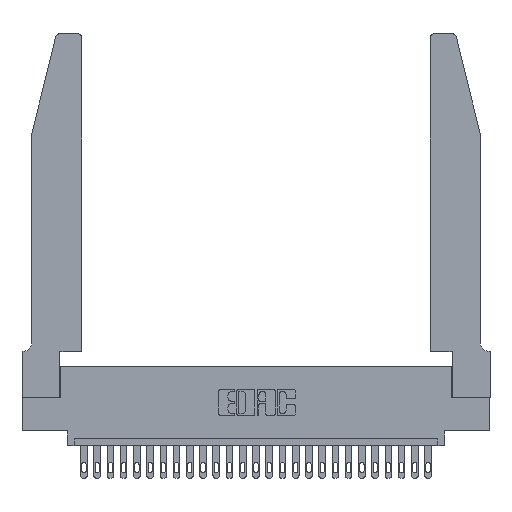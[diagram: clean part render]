
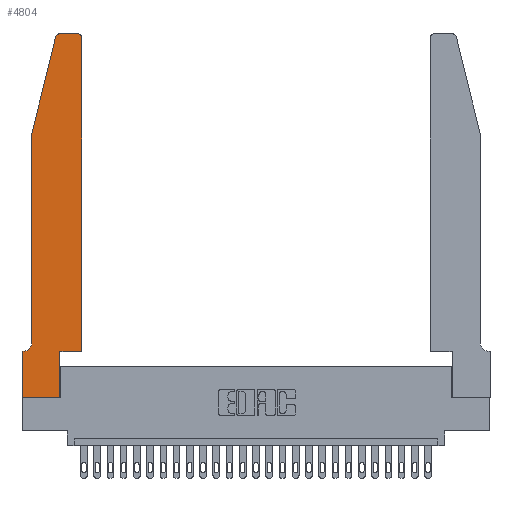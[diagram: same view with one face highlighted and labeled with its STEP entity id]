
A CAD part, top view. The second image highlights one B-rep face of the part: STEP entity #4804.
In plain terms, the highlighted planar face has unit normal (0, 0, 1).
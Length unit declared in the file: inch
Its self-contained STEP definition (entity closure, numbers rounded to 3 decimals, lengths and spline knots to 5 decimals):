
#257 = ORIENTED_EDGE ( 'NONE', *, *, #9147, .T. ) ;
#504 = VECTOR ( 'NONE', #16378, 39.37008 ) ;
#783 = DIRECTION ( 'NONE',  ( 0., 1., 0. ) ) ;
#1056 = DIRECTION ( 'NONE',  ( 0., 1., 0. ) ) ;
#1194 = FACE_OUTER_BOUND ( 'NONE', #2772, .T. ) ;
#1203 = CARTESIAN_POINT ( 'NONE',  ( 0.284, 2.75, 0.37 ) ) ;
#1291 = EDGE_CURVE ( 'NONE', #14044, #6601, #13889, .T. ) ;
#1710 = CARTESIAN_POINT ( 'NONE',  ( 0.4505, 0.35, 0.37 ) ) ;
#2290 = EDGE_CURVE ( 'NONE', #6111, #10012, #6612, .T. ) ;
#2717 = EDGE_CURVE ( 'NONE', #25058, #5606, #3269, .T. ) ;
#2722 = ORIENTED_EDGE ( 'NONE', *, *, #20206, .T. ) ;
#2772 = EDGE_LOOP ( 'NONE', ( #2722, #257, #8792, #23075, #24267, #3201, #9361, #20812, #14859, #9114, #6241, #6489 ) ) ;
#3201 = ORIENTED_EDGE ( 'NONE', *, *, #23624, .T. ) ;
#3269 = LINE ( 'NONE', #16344, #23928 ) ;
#3772 = DIRECTION ( 'NONE',  ( 1., 0., 0. ) ) ;
#4420 = DIRECTION ( 'NONE',  ( 1., 0., 0. ) ) ;
#4433 = LINE ( 'NONE', #26250, #20821 ) ;
#4804 = ADVANCED_FACE ( 'NONE', ( #1194 ), #10210, .T. ) ;
#5007 = LINE ( 'NONE', #11895, #7001 ) ;
#5606 = VERTEX_POINT ( 'NONE', #18691 ) ;
#6111 = VERTEX_POINT ( 'NONE', #23086 ) ;
#6241 = ORIENTED_EDGE ( 'NONE', *, *, #11447, .T. ) ;
#6354 = CARTESIAN_POINT ( 'NONE',  ( 0., 0.35, 0.37 ) ) ;
#6489 = ORIENTED_EDGE ( 'NONE', *, *, #8309, .T. ) ;
#6577 = VERTEX_POINT ( 'NONE', #1203 ) ;
#6601 = VERTEX_POINT ( 'NONE', #22659 ) ;
#6612 = LINE ( 'NONE', #17924, #26248 ) ;
#6940 = VERTEX_POINT ( 'NONE', #8079 ) ;
#7001 = VECTOR ( 'NONE', #11710, 39.37008 ) ;
#7949 = DIRECTION ( 'NONE',  ( 1., 0., 0. ) ) ;
#8079 = CARTESIAN_POINT ( 'NONE',  ( 0.4505, 2.72, 0.37 ) ) ;
#8309 = EDGE_CURVE ( 'NONE', #6940, #18835, #13226, .T. ) ;
#8479 = CARTESIAN_POINT ( 'NONE',  ( 0., 0., 0.37 ) ) ;
#8559 = CARTESIAN_POINT ( 'NONE',  ( 0.4505, 0.35, 0.37 ) ) ;
#8792 = ORIENTED_EDGE ( 'NONE', *, *, #22982, .T. ) ;
#9114 = ORIENTED_EDGE ( 'NONE', *, *, #10617, .T. ) ;
#9147 = EDGE_CURVE ( 'NONE', #6577, #14540, #26562, .T. ) ;
#9361 = ORIENTED_EDGE ( 'NONE', *, *, #2717, .T. ) ;
#9364 = DIRECTION ( 'NONE',  ( 0., -1., 0. ) ) ;
#10012 = VERTEX_POINT ( 'NONE', #26334 ) ;
#10025 = CARTESIAN_POINT ( 'NONE',  ( 0., 0.35, 0.37 ) ) ;
#10160 = CARTESIAN_POINT ( 'NONE',  ( 0.284, 2.72, 0.37 ) ) ;
#10210 = PLANE ( 'NONE',  #24173 ) ;
#10455 = EDGE_CURVE ( 'NONE', #6601, #27066, #18243, .T. ) ;
#10617 = EDGE_CURVE ( 'NONE', #10012, #19004, #22824, .T. ) ;
#11434 = CARTESIAN_POINT ( 'NONE',  ( 0.25487, 2.72718, 0.37 ) ) ;
#11447 = EDGE_CURVE ( 'NONE', #19004, #6940, #4433, .T. ) ;
#11710 = DIRECTION ( 'NONE',  ( -0.239, -0.971, 0. ) ) ;
#11895 = CARTESIAN_POINT ( 'NONE',  ( 0.0755, 2., 0.37 ) ) ;
#11947 = CARTESIAN_POINT ( 'NONE',  ( 0.0755, 0.35, 0.37 ) ) ;
#12189 = DIRECTION ( 'NONE',  ( 0., 0., 1. ) ) ;
#12270 = DIRECTION ( 'NONE',  ( 0., -1., 0. ) ) ;
#12609 = CARTESIAN_POINT ( 'NONE',  ( 0.4205, 2.75, 0.37 ) ) ;
#13226 = CIRCLE ( 'NONE', #17320, 0.03 ) ;
#13346 = CARTESIAN_POINT ( 'NONE',  ( 0.0755, 2., 0.37 ) ) ;
#13579 = CARTESIAN_POINT ( 'NONE',  ( 0.0755, 2., 0.37 ) ) ;
#13889 = LINE ( 'NONE', #13579, #21407 ) ;
#14044 = VERTEX_POINT ( 'NONE', #13346 ) ;
#14229 = LINE ( 'NONE', #8479, #19104 ) ;
#14540 = VERTEX_POINT ( 'NONE', #11434 ) ;
#14859 = ORIENTED_EDGE ( 'NONE', *, *, #2290, .T. ) ;
#15528 = DIRECTION ( 'NONE',  ( -1., 0., 0. ) ) ;
#16344 = CARTESIAN_POINT ( 'NONE',  ( 0., 0., 0.37 ) ) ;
#16378 = DIRECTION ( 'NONE',  ( 1., 0., 0. ) ) ;
#17320 = AXIS2_PLACEMENT_3D ( 'NONE', #18949, #21153, #18783 ) ;
#17924 = CARTESIAN_POINT ( 'NONE',  ( 0.2865, 0.35, 0.37 ) ) ;
#18243 = CIRCLE ( 'NONE', #24361, 0.07 ) ;
#18691 = CARTESIAN_POINT ( 'NONE',  ( 0., 0., 0.37 ) ) ;
#18763 = CARTESIAN_POINT ( 'NONE',  ( 0.0055, 0.35, 0.37 ) ) ;
#18783 = DIRECTION ( 'NONE',  ( 1., 0., 0. ) ) ;
#18835 = VERTEX_POINT ( 'NONE', #12609 ) ;
#18949 = CARTESIAN_POINT ( 'NONE',  ( 0.4205, 2.72, 0.37 ) ) ;
#19004 = VERTEX_POINT ( 'NONE', #8559 ) ;
#19104 = VECTOR ( 'NONE', #4420, 39.37008 ) ;
#19816 = CARTESIAN_POINT ( 'NONE',  ( 0.2605, 2.75, 0.37 ) ) ;
#20206 = EDGE_CURVE ( 'NONE', #18835, #6577, #25674, .T. ) ;
#20812 = ORIENTED_EDGE ( 'NONE', *, *, #21458, .T. ) ;
#20821 = VECTOR ( 'NONE', #783, 39.37008 ) ;
#21153 = DIRECTION ( 'NONE',  ( 0., 0., 1. ) ) ;
#21250 = CARTESIAN_POINT ( 'NONE',  ( 0.0055, 0.42, 0.37 ) ) ;
#21341 = DIRECTION ( 'NONE',  ( -1., 0., 0. ) ) ;
#21407 = VECTOR ( 'NONE', #9364, 39.37008 ) ;
#21458 = EDGE_CURVE ( 'NONE', #5606, #6111, #14229, .T. ) ;
#22522 = DIRECTION ( 'NONE',  ( -1., 0., 0. ) ) ;
#22659 = CARTESIAN_POINT ( 'NONE',  ( 0.0755, 0.42, 0.37 ) ) ;
#22824 = LINE ( 'NONE', #1710, #504 ) ;
#22982 = EDGE_CURVE ( 'NONE', #14540, #14044, #5007, .T. ) ;
#23075 = ORIENTED_EDGE ( 'NONE', *, *, #1291, .T. ) ;
#23081 = VECTOR ( 'NONE', #15528, 39.37008 ) ;
#23086 = CARTESIAN_POINT ( 'NONE',  ( 0.2865, 0., 0.37 ) ) ;
#23299 = AXIS2_PLACEMENT_3D ( 'NONE', #10160, #12189, #7949 ) ;
#23624 = EDGE_CURVE ( 'NONE', #27066, #25058, #26947, .T. ) ;
#23928 = VECTOR ( 'NONE', #12270, 39.37008 ) ;
#24173 = AXIS2_PLACEMENT_3D ( 'NONE', #10025, #24819, #3772 ) ;
#24267 = ORIENTED_EDGE ( 'NONE', *, *, #10455, .T. ) ;
#24361 = AXIS2_PLACEMENT_3D ( 'NONE', #21250, #25794, #21341 ) ;
#24819 = DIRECTION ( 'NONE',  ( 0., 0., 1. ) ) ;
#25058 = VERTEX_POINT ( 'NONE', #6354 ) ;
#25674 = LINE ( 'NONE', #19816, #23081 ) ;
#25794 = DIRECTION ( 'NONE',  ( 0., 0., -1. ) ) ;
#26248 = VECTOR ( 'NONE', #1056, 39.37008 ) ;
#26250 = CARTESIAN_POINT ( 'NONE',  ( 0.4505, 0.35, 0.37 ) ) ;
#26264 = VECTOR ( 'NONE', #22522, 39.37008 ) ;
#26334 = CARTESIAN_POINT ( 'NONE',  ( 0.2865, 0.35, 0.37 ) ) ;
#26562 = CIRCLE ( 'NONE', #23299, 0.03 ) ;
#26947 = LINE ( 'NONE', #11947, #26264 ) ;
#27066 = VERTEX_POINT ( 'NONE', #18763 ) ;
